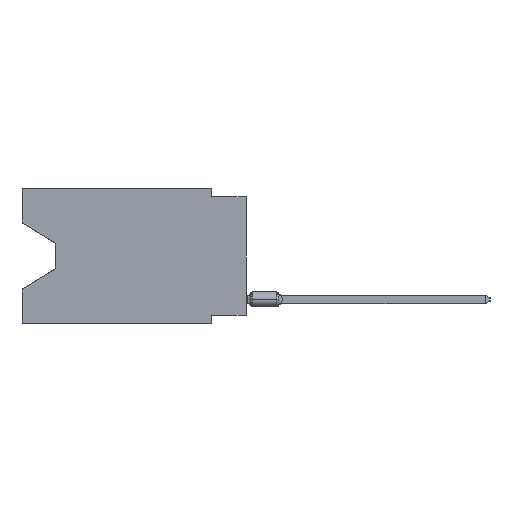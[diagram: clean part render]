
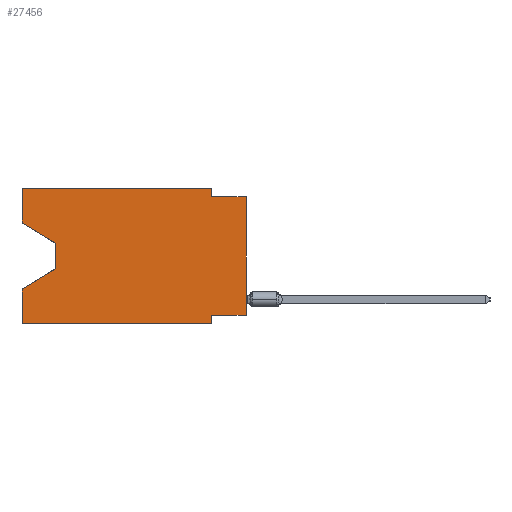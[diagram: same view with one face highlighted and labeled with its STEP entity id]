
A CAD part, left-side view. The second image highlights one B-rep face of the part: STEP entity #27456.
In plain terms, the highlighted planar face has unit normal (-1, 0, 0).
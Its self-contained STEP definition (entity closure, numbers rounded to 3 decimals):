
#710 = CARTESIAN_POINT ( 'NONE',  ( 0., 2.54, -0.635 ) ) ;
#990 = CARTESIAN_POINT ( 'NONE',  ( 0., 16.383, 0. ) ) ;
#2169 = DIRECTION ( 'NONE',  ( 0., 0., 1. ) ) ;
#4944 = CARTESIAN_POINT ( 'NONE',  ( 0., 13.97, -4.013 ) ) ;
#8175 = CARTESIAN_POINT ( 'NONE',  ( 0., 16.383, 0. ) ) ;
#9659 = DIRECTION ( 'NONE',  ( 0., 0., 1. ) ) ;
#10930 = DIRECTION ( 'NONE',  ( 1., 0., 0. ) ) ;
#11222 = ORIENTED_EDGE ( 'NONE', *, *, #68220, .F. ) ;
#13627 = VERTEX_POINT ( 'NONE', #25468 ) ;
#13631 = EDGE_CURVE ( 'NONE', #44863, #66352, #48448, .T. ) ;
#14028 = EDGE_CURVE ( 'NONE', #34808, #21151, #20002, .T. ) ;
#14351 = EDGE_CURVE ( 'NONE', #38479, #34808, #66945, .T. ) ;
#14456 = CARTESIAN_POINT ( 'NONE',  ( 0., 13.97, -4.013 ) ) ;
#14713 = CARTESIAN_POINT ( 'NONE',  ( 0., 0., -0.635 ) ) ;
#14722 = LINE ( 'NONE', #20742, #47479 ) ;
#14816 = DIRECTION ( 'NONE',  ( 0., 0., -1. ) ) ;
#14829 = ORIENTED_EDGE ( 'NONE', *, *, #70370, .T. ) ;
#14962 = ORIENTED_EDGE ( 'NONE', *, *, #51064, .F. ) ;
#16774 = DIRECTION ( 'NONE',  ( 0., 0., 1. ) ) ;
#16804 = DIRECTION ( 'NONE',  ( 0., -1., 0. ) ) ;
#17088 = DIRECTION ( 'NONE',  ( 0., 1., 0. ) ) ;
#17299 = ORIENTED_EDGE ( 'NONE', *, *, #48832, .T. ) ;
#18080 = EDGE_CURVE ( 'NONE', #64864, #63179, #52353, .T. ) ;
#18824 = VECTOR ( 'NONE', #14816, 1000. ) ;
#20002 = LINE ( 'NONE', #14713, #61570 ) ;
#20742 = CARTESIAN_POINT ( 'NONE',  ( 0., 16.383, -2.546 ) ) ;
#21151 = VERTEX_POINT ( 'NONE', #36018 ) ;
#23947 = LINE ( 'NONE', #990, #44430 ) ;
#24098 = ORIENTED_EDGE ( 'NONE', *, *, #28384, .F. ) ;
#25297 = VERTEX_POINT ( 'NONE', #60367 ) ;
#25468 = CARTESIAN_POINT ( 'NONE',  ( 0., 16.383, -9.906 ) ) ;
#27427 = EDGE_CURVE ( 'NONE', #74083, #34217, #14722, .T. ) ;
#27444 = CARTESIAN_POINT ( 'NONE',  ( 0., 16.383, -7.36 ) ) ;
#27456 = ADVANCED_FACE ( 'NONE', ( #36973 ), #68161, .F. ) ;
#28135 = VECTOR ( 'NONE', #48919, 1000. ) ;
#28384 = EDGE_CURVE ( 'NONE', #13627, #66352, #68355, .T. ) ;
#28453 = CARTESIAN_POINT ( 'NONE',  ( 0., 16.383, -9.906 ) ) ;
#34217 = VERTEX_POINT ( 'NONE', #4944 ) ;
#34808 = VERTEX_POINT ( 'NONE', #710 ) ;
#34919 = ORIENTED_EDGE ( 'NONE', *, *, #48632, .T. ) ;
#35008 = CARTESIAN_POINT ( 'NONE',  ( 0., 0., -9.271 ) ) ;
#36018 = CARTESIAN_POINT ( 'NONE',  ( 0., 0., -0.635 ) ) ;
#36357 = CARTESIAN_POINT ( 'NONE',  ( 0., 2.54, 0. ) ) ;
#36973 = FACE_OUTER_BOUND ( 'NONE', #42563, .T. ) ;
#37693 = DIRECTION ( 'NONE',  ( 0., -1., 0. ) ) ;
#37925 = ORIENTED_EDGE ( 'NONE', *, *, #14028, .F. ) ;
#38479 = VERTEX_POINT ( 'NONE', #36357 ) ;
#40826 = CARTESIAN_POINT ( 'NONE',  ( 0., 0., -9.271 ) ) ;
#41062 = CARTESIAN_POINT ( 'NONE',  ( 0., 2.54, -9.271 ) ) ;
#41106 = CARTESIAN_POINT ( 'NONE',  ( 0., 13.97, -5.893 ) ) ;
#41726 = LINE ( 'NONE', #8175, #48104 ) ;
#42563 = EDGE_LOOP ( 'NONE', ( #58381, #17299, #61063, #24098, #34919, #44440, #14962, #14829, #37925, #68956, #11222, #46553 ) ) ;
#42729 = VECTOR ( 'NONE', #16774, 1000. ) ;
#44430 = VECTOR ( 'NONE', #16804, 1000. ) ;
#44440 = ORIENTED_EDGE ( 'NONE', *, *, #18080, .F. ) ;
#44863 = VERTEX_POINT ( 'NONE', #41106 ) ;
#46553 = ORIENTED_EDGE ( 'NONE', *, *, #66620, .F. ) ;
#46846 = VERTEX_POINT ( 'NONE', #35008 ) ;
#47479 = VECTOR ( 'NONE', #72701, 1000. ) ;
#48104 = VECTOR ( 'NONE', #2169, 1000. ) ;
#48448 = LINE ( 'NONE', #71396, #63894 ) ;
#48632 = EDGE_CURVE ( 'NONE', #13627, #63179, #66860, .T. ) ;
#48780 = VECTOR ( 'NONE', #51242, 1000. ) ;
#48832 = EDGE_CURVE ( 'NONE', #34217, #44863, #60381, .T. ) ;
#48919 = DIRECTION ( 'NONE',  ( 0., 0., -1. ) ) ;
#49645 = CARTESIAN_POINT ( 'NONE',  ( 0., 2.54, 0. ) ) ;
#51064 = EDGE_CURVE ( 'NONE', #46846, #64864, #68672, .T. ) ;
#51242 = DIRECTION ( 'NONE',  ( 0., 0., -1. ) ) ;
#52353 = LINE ( 'NONE', #63257, #48780 ) ;
#56337 = CARTESIAN_POINT ( 'NONE',  ( 0., 0., 0. ) ) ;
#56862 = DIRECTION ( 'NONE',  ( 0., 0., -1. ) ) ;
#58381 = ORIENTED_EDGE ( 'NONE', *, *, #27427, .T. ) ;
#60264 = VECTOR ( 'NONE', #9659, 1000. ) ;
#60367 = CARTESIAN_POINT ( 'NONE',  ( 0., 16.383, 0. ) ) ;
#60381 = LINE ( 'NONE', #14456, #18824 ) ;
#60459 = DIRECTION ( 'NONE',  ( 0., 0.855, -0.519 ) ) ;
#61063 = ORIENTED_EDGE ( 'NONE', *, *, #13631, .T. ) ;
#61570 = VECTOR ( 'NONE', #37693, 1000. ) ;
#62507 = CARTESIAN_POINT ( 'NONE',  ( 0., 16.383, 0. ) ) ;
#63179 = VERTEX_POINT ( 'NONE', #70937 ) ;
#63257 = CARTESIAN_POINT ( 'NONE',  ( 0., 2.54, -9.906 ) ) ;
#63265 = VECTOR ( 'NONE', #68353, 1000. ) ;
#63894 = VECTOR ( 'NONE', #60459, 1000. ) ;
#64864 = VERTEX_POINT ( 'NONE', #41062 ) ;
#66352 = VERTEX_POINT ( 'NONE', #27444 ) ;
#66620 = EDGE_CURVE ( 'NONE', #74083, #25297, #41726, .T. ) ;
#66860 = LINE ( 'NONE', #28453, #63265 ) ;
#66945 = LINE ( 'NONE', #49645, #28135 ) ;
#68161 = PLANE ( 'NONE',  #73938 ) ;
#68220 = EDGE_CURVE ( 'NONE', #25297, #38479, #23947, .T. ) ;
#68353 = DIRECTION ( 'NONE',  ( 0., -1., 0. ) ) ;
#68355 = LINE ( 'NONE', #72892, #42729 ) ;
#68672 = LINE ( 'NONE', #40826, #71716 ) ;
#68956 = ORIENTED_EDGE ( 'NONE', *, *, #14351, .F. ) ;
#70370 = EDGE_CURVE ( 'NONE', #46846, #21151, #73283, .T. ) ;
#70937 = CARTESIAN_POINT ( 'NONE',  ( 0., 2.54, -9.906 ) ) ;
#71396 = CARTESIAN_POINT ( 'NONE',  ( 0., 13.97, -5.893 ) ) ;
#71716 = VECTOR ( 'NONE', #17088, 1000. ) ;
#71955 = CARTESIAN_POINT ( 'NONE',  ( 0., 16.383, -2.546 ) ) ;
#72701 = DIRECTION ( 'NONE',  ( 0., -0.855, -0.519 ) ) ;
#72892 = CARTESIAN_POINT ( 'NONE',  ( 0., 16.383, 0. ) ) ;
#73283 = LINE ( 'NONE', #56337, #60264 ) ;
#73938 = AXIS2_PLACEMENT_3D ( 'NONE', #62507, #10930, #56862 ) ;
#74083 = VERTEX_POINT ( 'NONE', #71955 ) ;
